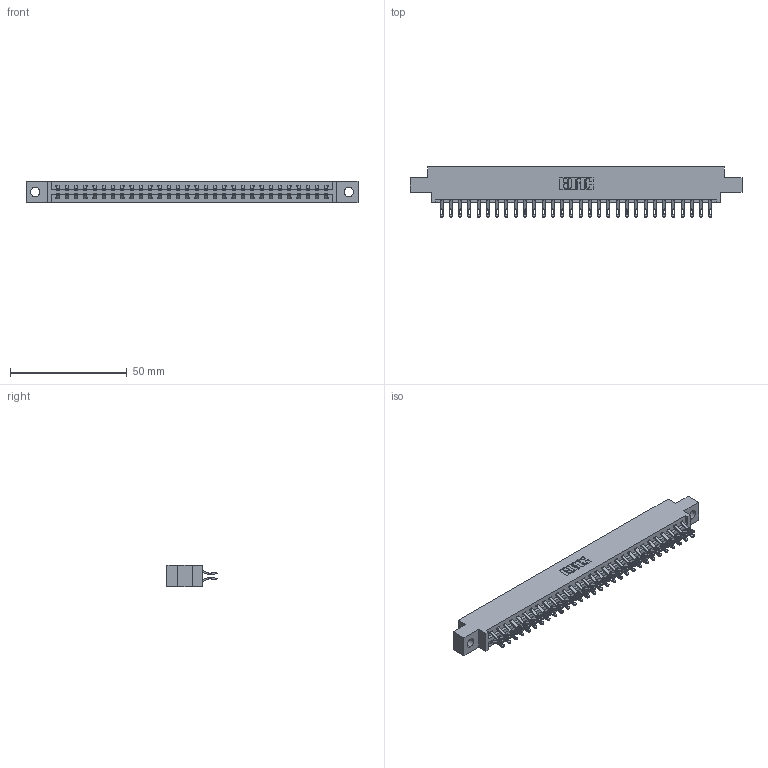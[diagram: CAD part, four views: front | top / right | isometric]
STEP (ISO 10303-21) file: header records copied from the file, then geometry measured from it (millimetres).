
FILE_DESCRIPTION (( 'STEP AP203' ), '1' );
FILE_NAME ('387-060-555-804.STEP', '2018-09-21T03:51:47', ( '' ), ( '' ), 'SwSTEP 2.0', 'SolidWorks 2016', '' );
FILE_SCHEMA (( 'CONFIG_CONTROL_DESIGN' ));
Length unit declared in the file: inch
Products named in the file (3): 337 Part_0.170 Offset - 0.156 Dia-TH; 345-292-001_555 Tail; 387-060-555-804
Assembly tree (61 placements, depth 2):
  387-060-555-804
    337 Part_0.170 Offset - 0.156 Dia-TH
    345-292-001_555 Tail  x60
Bounding box: 141.88 x 21.47 x 9.4 mm (x, y, z)
Volume: 14761.8 mm3; surface area: 17132.8 mm2
Topology: 61 solids, 61 shells, 3718 faces, 11663 edges, 7774 vertices
Faces by surface type: plane 2234, cylinder 1484
Entity records: 25273 total; most frequent: CARTESIAN_POINT 4304, ORIENTED_EDGE 4210, DIRECTION 3653, EDGE_CURVE 2105, VECTOR 1957, LINE 1957, VERTEX_POINT 1402, AXIS2_PLACEMENT_3D 848
